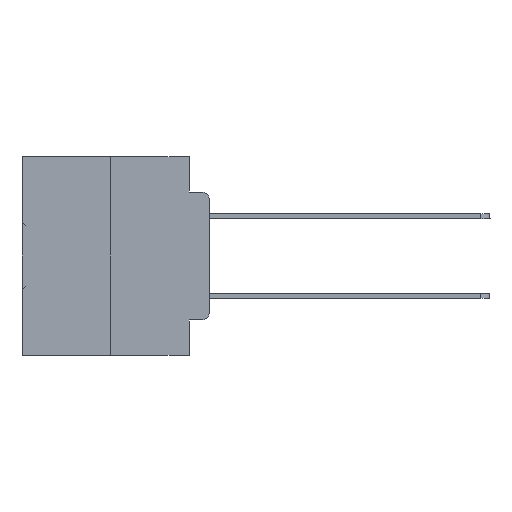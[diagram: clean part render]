
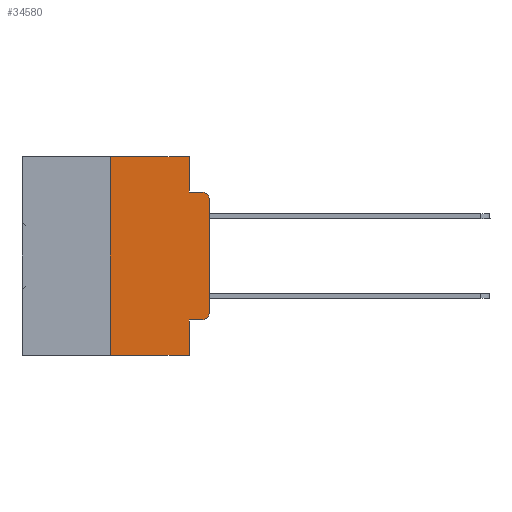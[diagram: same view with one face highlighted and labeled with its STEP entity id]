
A CAD part, left-side view. The second image highlights one B-rep face of the part: STEP entity #34580.
In plain terms, the highlighted planar face has unit normal (-1, 0, 0).
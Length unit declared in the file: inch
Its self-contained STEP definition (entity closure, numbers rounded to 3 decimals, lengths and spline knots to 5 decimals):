
#10 = VERTEX_POINT ( 'NONE', #22239 ) ;
#168 = CARTESIAN_POINT ( 'NONE',  ( 0., 0.051, 0. ) ) ;
#969 = CARTESIAN_POINT ( 'NONE',  ( 0., 0.473, -0.5 ) ) ;
#1319 = ORIENTED_EDGE ( 'NONE', *, *, #32103, .F. ) ;
#2519 = VECTOR ( 'NONE', #23225, 39.37008 ) ;
#3028 = CARTESIAN_POINT ( 'NONE',  ( 0., 0.02, -0.0885 ) ) ;
#3274 = DIRECTION ( 'NONE',  ( 0., 0., -1. ) ) ;
#3848 = CARTESIAN_POINT ( 'NONE',  ( 0., 0.051, 0. ) ) ;
#4815 = EDGE_CURVE ( 'NONE', #15651, #23799, #7125, .T. ) ;
#5058 = DIRECTION ( 'NONE',  ( 0., 0., -1. ) ) ;
#5076 = ORIENTED_EDGE ( 'NONE', *, *, #7623, .F. ) ;
#5510 = LINE ( 'NONE', #32281, #9778 ) ;
#6537 = EDGE_CURVE ( 'NONE', #12455, #20898, #34863, .T. ) ;
#7125 = LINE ( 'NONE', #32973, #35411 ) ;
#7593 = ORIENTED_EDGE ( 'NONE', *, *, #26883, .F. ) ;
#7623 = EDGE_CURVE ( 'NONE', #15651, #20719, #28793, .T. ) ;
#7843 = VECTOR ( 'NONE', #5058, 39.37008 ) ;
#8881 = CARTESIAN_POINT ( 'NONE',  ( 0., 0., 0. ) ) ;
#9231 = LINE ( 'NONE', #8881, #16911 ) ;
#9565 = DIRECTION ( 'NONE',  ( 0., -1., 0. ) ) ;
#9603 = EDGE_CURVE ( 'NONE', #10, #20719, #20929, .T. ) ;
#9778 = VECTOR ( 'NONE', #29985, 39.37008 ) ;
#9830 = CARTESIAN_POINT ( 'NONE',  ( 0., 0.051, -0.0885 ) ) ;
#10381 = DIRECTION ( 'NONE',  ( 0., 0., -1. ) ) ;
#11045 = EDGE_CURVE ( 'NONE', #13130, #20567, #9231, .T. ) ;
#11471 = LINE ( 'NONE', #14931, #2519 ) ;
#12394 = CARTESIAN_POINT ( 'NONE',  ( 0., 0.02, -0.3915 ) ) ;
#12455 = VERTEX_POINT ( 'NONE', #21354 ) ;
#12899 = LINE ( 'NONE', #168, #7843 ) ;
#13130 = VERTEX_POINT ( 'NONE', #34757 ) ;
#13189 = ORIENTED_EDGE ( 'NONE', *, *, #11045, .T. ) ;
#14445 = ORIENTED_EDGE ( 'NONE', *, *, #6537, .F. ) ;
#14931 = CARTESIAN_POINT ( 'NONE',  ( 0., 0.473, 0. ) ) ;
#15483 = VERTEX_POINT ( 'NONE', #26299 ) ;
#15651 = VERTEX_POINT ( 'NONE', #34021 ) ;
#16470 = CARTESIAN_POINT ( 'NONE',  ( 0., 0.473, 0. ) ) ;
#16610 = DIRECTION ( 'NONE',  ( 0., -1., 0. ) ) ;
#16911 = VECTOR ( 'NONE', #19513, 39.37008 ) ;
#17648 = CARTESIAN_POINT ( 'NONE',  ( 0., 0.02, -0.4115 ) ) ;
#17946 = DIRECTION ( 'NONE',  ( 0., -1., 0. ) ) ;
#18628 = DIRECTION ( 'NONE',  ( -1., 0., 0. ) ) ;
#18828 = ORIENTED_EDGE ( 'NONE', *, *, #28549, .T. ) ;
#19472 = DIRECTION ( 'NONE',  ( 1., 0., 0. ) ) ;
#19513 = DIRECTION ( 'NONE',  ( 0., 0., 1. ) ) ;
#20330 = CIRCLE ( 'NONE', #24194, 0.02 ) ;
#20567 = VERTEX_POINT ( 'NONE', #24978 ) ;
#20719 = VERTEX_POINT ( 'NONE', #29974 ) ;
#20898 = VERTEX_POINT ( 'NONE', #3028 ) ;
#20929 = LINE ( 'NONE', #969, #26976 ) ;
#21001 = ORIENTED_EDGE ( 'NONE', *, *, #9603, .T. ) ;
#21202 = EDGE_LOOP ( 'NONE', ( #13189, #18828, #14445, #23620, #7593, #1319, #21001, #5076, #33612, #26809 ) ) ;
#21354 = CARTESIAN_POINT ( 'NONE',  ( 0., 0.051, -0.0885 ) ) ;
#21532 = VECTOR ( 'NONE', #17946, 39.37008 ) ;
#22239 = CARTESIAN_POINT ( 'NONE',  ( 0., 0.25, -0.5 ) ) ;
#22737 = DIRECTION ( 'NONE',  ( -1., 0., 0. ) ) ;
#23225 = DIRECTION ( 'NONE',  ( 0., -1., 0. ) ) ;
#23620 = ORIENTED_EDGE ( 'NONE', *, *, #30260, .F. ) ;
#23799 = VERTEX_POINT ( 'NONE', #17648 ) ;
#23821 = FACE_OUTER_BOUND ( 'NONE', #21202, .T. ) ;
#24194 = AXIS2_PLACEMENT_3D ( 'NONE', #33554, #22737, #3274 ) ;
#24290 = CIRCLE ( 'NONE', #32452, 0.02 ) ;
#24978 = CARTESIAN_POINT ( 'NONE',  ( 0., 0., -0.1085 ) ) ;
#25317 = VERTEX_POINT ( 'NONE', #29815 ) ;
#25893 = DIRECTION ( 'NONE',  ( 0., 0., -1. ) ) ;
#26217 = VECTOR ( 'NONE', #25893, 39.37008 ) ;
#26299 = CARTESIAN_POINT ( 'NONE',  ( 0., 0.25, 0. ) ) ;
#26809 = ORIENTED_EDGE ( 'NONE', *, *, #27506, .T. ) ;
#26883 = EDGE_CURVE ( 'NONE', #15483, #25317, #11471, .T. ) ;
#26976 = VECTOR ( 'NONE', #9565, 39.37008 ) ;
#27506 = EDGE_CURVE ( 'NONE', #23799, #13130, #24290, .T. ) ;
#27573 = DIRECTION ( 'NONE',  ( 0., 0., -1. ) ) ;
#28549 = EDGE_CURVE ( 'NONE', #20567, #20898, #20330, .T. ) ;
#28793 = LINE ( 'NONE', #3848, #26217 ) ;
#29815 = CARTESIAN_POINT ( 'NONE',  ( 0., 0.051, 0. ) ) ;
#29974 = CARTESIAN_POINT ( 'NONE',  ( 0., 0.051, -0.5 ) ) ;
#29985 = DIRECTION ( 'NONE',  ( 0., 0., 1. ) ) ;
#30260 = EDGE_CURVE ( 'NONE', #25317, #12455, #12899, .T. ) ;
#31219 = AXIS2_PLACEMENT_3D ( 'NONE', #16470, #19472, #27573 ) ;
#31238 = PLANE ( 'NONE',  #31219 ) ;
#32103 = EDGE_CURVE ( 'NONE', #10, #15483, #5510, .T. ) ;
#32281 = CARTESIAN_POINT ( 'NONE',  ( 0., 0.25, 0. ) ) ;
#32452 = AXIS2_PLACEMENT_3D ( 'NONE', #12394, #18628, #10381 ) ;
#32973 = CARTESIAN_POINT ( 'NONE',  ( 0., 0.051, -0.4115 ) ) ;
#33554 = CARTESIAN_POINT ( 'NONE',  ( 0., 0.02, -0.1085 ) ) ;
#33612 = ORIENTED_EDGE ( 'NONE', *, *, #4815, .T. ) ;
#34021 = CARTESIAN_POINT ( 'NONE',  ( 0., 0.051, -0.4115 ) ) ;
#34580 = ADVANCED_FACE ( 'NONE', ( #23821 ), #31238, .F. ) ;
#34757 = CARTESIAN_POINT ( 'NONE',  ( 0., 0., -0.3915 ) ) ;
#34863 = LINE ( 'NONE', #9830, #21532 ) ;
#35411 = VECTOR ( 'NONE', #16610, 39.37008 ) ;
